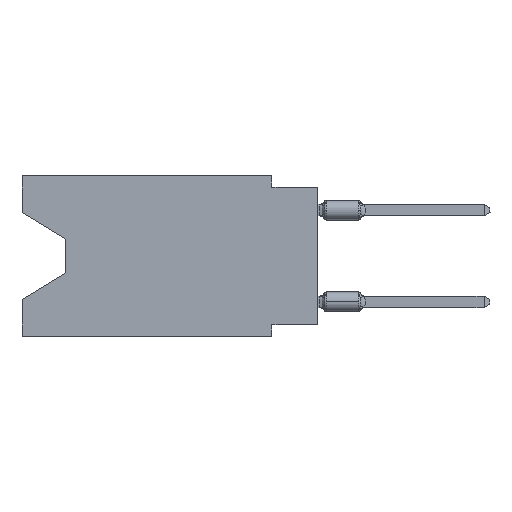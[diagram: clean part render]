
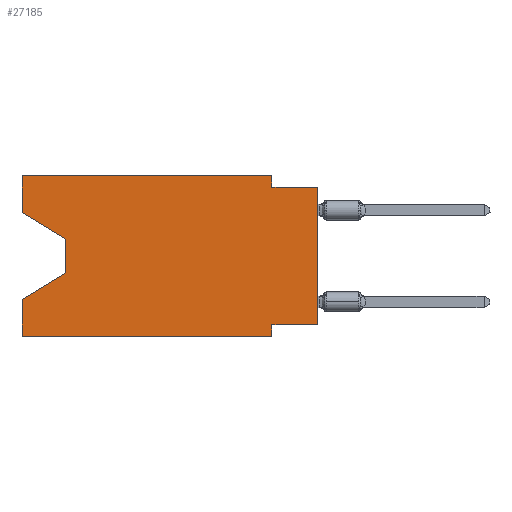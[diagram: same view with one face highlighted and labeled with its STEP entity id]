
A CAD part, left-side view. The second image highlights one B-rep face of the part: STEP entity #27185.
In plain terms, the highlighted planar face has unit normal (-1, 0, 0).
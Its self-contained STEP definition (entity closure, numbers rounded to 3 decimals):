
#173 = ORIENTED_EDGE ( 'NONE', *, *, #14531, .T. ) ;
#1053 = CARTESIAN_POINT ( 'NONE',  ( 0., 2.54, 0. ) ) ;
#1490 = CARTESIAN_POINT ( 'NONE',  ( 0., 16.383, -8.89 ) ) ;
#1505 = DIRECTION ( 'NONE',  ( 0., -1., 0. ) ) ;
#1600 = VERTEX_POINT ( 'NONE', #3688 ) ;
#1727 = ORIENTED_EDGE ( 'NONE', *, *, #35090, .T. ) ;
#1918 = CARTESIAN_POINT ( 'NONE',  ( 0., 2.54, -8.255 ) ) ;
#2110 = VERTEX_POINT ( 'NONE', #28559 ) ;
#2384 = VECTOR ( 'NONE', #1505, 1000. ) ;
#2463 = CARTESIAN_POINT ( 'NONE',  ( 0., 13.97, -5.385 ) ) ;
#3688 = CARTESIAN_POINT ( 'NONE',  ( 0., 13.97, -5.385 ) ) ;
#3735 = CARTESIAN_POINT ( 'NONE',  ( 0., 0., -0.635 ) ) ;
#5222 = LINE ( 'NONE', #19776, #11342 ) ;
#6176 = CARTESIAN_POINT ( 'NONE',  ( 0., 16.383, 0. ) ) ;
#6453 = VERTEX_POINT ( 'NONE', #34848 ) ;
#6454 = LINE ( 'NONE', #29892, #19715 ) ;
#6545 = DIRECTION ( 'NONE',  ( 0., 0., -1. ) ) ;
#6986 = ORIENTED_EDGE ( 'NONE', *, *, #32904, .F. ) ;
#8345 = VECTOR ( 'NONE', #33208, 1000. ) ;
#11218 = PLANE ( 'NONE',  #14468 ) ;
#11342 = VECTOR ( 'NONE', #28472, 1000. ) ;
#11491 = EDGE_CURVE ( 'NONE', #31974, #31664, #28038, .T. ) ;
#11546 = ORIENTED_EDGE ( 'NONE', *, *, #26068, .F. ) ;
#11664 = DIRECTION ( 'NONE',  ( 0., -1., 0. ) ) ;
#12173 = VERTEX_POINT ( 'NONE', #15195 ) ;
#12175 = CARTESIAN_POINT ( 'NONE',  ( 0., 2.54, -8.89 ) ) ;
#12543 = LINE ( 'NONE', #18385, #14503 ) ;
#13282 = DIRECTION ( 'NONE',  ( 0., 0., 1. ) ) ;
#13915 = VECTOR ( 'NONE', #13282, 1000. ) ;
#14278 = LINE ( 'NONE', #34992, #37591 ) ;
#14468 = AXIS2_PLACEMENT_3D ( 'NONE', #6176, #23044, #34839 ) ;
#14503 = VECTOR ( 'NONE', #6545, 1000. ) ;
#14531 = EDGE_CURVE ( 'NONE', #6453, #1600, #14278, .T. ) ;
#14732 = ORIENTED_EDGE ( 'NONE', *, *, #16717, .F. ) ;
#15039 = EDGE_CURVE ( 'NONE', #15574, #6453, #6454, .T. ) ;
#15195 = CARTESIAN_POINT ( 'NONE',  ( 0., 16.383, 0. ) ) ;
#15276 = LINE ( 'NONE', #16893, #19425 ) ;
#15574 = VERTEX_POINT ( 'NONE', #21343 ) ;
#15606 = DIRECTION ( 'NONE',  ( 0., 1., 0. ) ) ;
#16452 = ORIENTED_EDGE ( 'NONE', *, *, #33744, .F. ) ;
#16717 = EDGE_CURVE ( 'NONE', #12173, #18472, #32379, .T. ) ;
#16893 = CARTESIAN_POINT ( 'NONE',  ( 0., 0., -0.635 ) ) ;
#16964 = VECTOR ( 'NONE', #26086, 1000. ) ;
#17087 = VERTEX_POINT ( 'NONE', #25392 ) ;
#17481 = ORIENTED_EDGE ( 'NONE', *, *, #28936, .F. ) ;
#18075 = VECTOR ( 'NONE', #11664, 1000. ) ;
#18157 = CARTESIAN_POINT ( 'NONE',  ( 0., 0., -8.255 ) ) ;
#18254 = CARTESIAN_POINT ( 'NONE',  ( 0., 16.383, 0. ) ) ;
#18385 = CARTESIAN_POINT ( 'NONE',  ( 0., 2.54, -8.89 ) ) ;
#18472 = VERTEX_POINT ( 'NONE', #37056 ) ;
#19158 = CARTESIAN_POINT ( 'NONE',  ( 0., 16.383, -8.89 ) ) ;
#19425 = VECTOR ( 'NONE', #29795, 1000. ) ;
#19715 = VECTOR ( 'NONE', #32229, 1000. ) ;
#19776 = CARTESIAN_POINT ( 'NONE',  ( 0., 16.383, 0. ) ) ;
#21069 = LINE ( 'NONE', #18157, #28153 ) ;
#21343 = CARTESIAN_POINT ( 'NONE',  ( 0., 16.383, -2.038 ) ) ;
#21698 = ORIENTED_EDGE ( 'NONE', *, *, #27615, .T. ) ;
#21775 = LINE ( 'NONE', #1053, #8345 ) ;
#21845 = EDGE_CURVE ( 'NONE', #18472, #29876, #21775, .T. ) ;
#23044 = DIRECTION ( 'NONE',  ( 1., 0., 0. ) ) ;
#25213 = EDGE_CURVE ( 'NONE', #15574, #12173, #5222, .T. ) ;
#25392 = CARTESIAN_POINT ( 'NONE',  ( 0., 16.383, -6.852 ) ) ;
#25735 = LINE ( 'NONE', #28824, #30532 ) ;
#26068 = EDGE_CURVE ( 'NONE', #36453, #31664, #12543, .T. ) ;
#26086 = DIRECTION ( 'NONE',  ( 0., 0.855, -0.519 ) ) ;
#27185 = ADVANCED_FACE ( 'NONE', ( #32716 ), #11218, .F. ) ;
#27615 = EDGE_CURVE ( 'NONE', #1600, #17087, #31902, .T. ) ;
#27989 = CARTESIAN_POINT ( 'NONE',  ( 0., 16.383, 0. ) ) ;
#28038 = LINE ( 'NONE', #19158, #2384 ) ;
#28153 = VECTOR ( 'NONE', #15606, 1000. ) ;
#28188 = LINE ( 'NONE', #27989, #13915 ) ;
#28472 = DIRECTION ( 'NONE',  ( 0., 0., 1. ) ) ;
#28559 = CARTESIAN_POINT ( 'NONE',  ( 0., 0., -8.255 ) ) ;
#28719 = ORIENTED_EDGE ( 'NONE', *, *, #11491, .T. ) ;
#28824 = CARTESIAN_POINT ( 'NONE',  ( 0., 0., 0. ) ) ;
#28936 = EDGE_CURVE ( 'NONE', #2110, #36453, #21069, .T. ) ;
#29012 = DIRECTION ( 'NONE',  ( 0., 0., 1. ) ) ;
#29758 = EDGE_LOOP ( 'NONE', ( #30259, #173, #21698, #16452, #28719, #11546, #17481, #1727, #6986, #29855, #14732, #34719 ) ) ;
#29795 = DIRECTION ( 'NONE',  ( 0., -1., 0. ) ) ;
#29855 = ORIENTED_EDGE ( 'NONE', *, *, #21845, .F. ) ;
#29876 = VERTEX_POINT ( 'NONE', #37578 ) ;
#29892 = CARTESIAN_POINT ( 'NONE',  ( 0., 16.383, -2.038 ) ) ;
#30259 = ORIENTED_EDGE ( 'NONE', *, *, #15039, .T. ) ;
#30532 = VECTOR ( 'NONE', #29012, 1000. ) ;
#31664 = VERTEX_POINT ( 'NONE', #12175 ) ;
#31902 = LINE ( 'NONE', #2463, #16964 ) ;
#31974 = VERTEX_POINT ( 'NONE', #1490 ) ;
#32229 = DIRECTION ( 'NONE',  ( 0., -0.855, -0.519 ) ) ;
#32379 = LINE ( 'NONE', #18254, #18075 ) ;
#32644 = VERTEX_POINT ( 'NONE', #3735 ) ;
#32716 = FACE_OUTER_BOUND ( 'NONE', #29758, .T. ) ;
#32904 = EDGE_CURVE ( 'NONE', #29876, #32644, #15276, .T. ) ;
#33208 = DIRECTION ( 'NONE',  ( 0., 0., -1. ) ) ;
#33744 = EDGE_CURVE ( 'NONE', #31974, #17087, #28188, .T. ) ;
#34719 = ORIENTED_EDGE ( 'NONE', *, *, #25213, .F. ) ;
#34839 = DIRECTION ( 'NONE',  ( 0., 0., -1. ) ) ;
#34848 = CARTESIAN_POINT ( 'NONE',  ( 0., 13.97, -3.505 ) ) ;
#34992 = CARTESIAN_POINT ( 'NONE',  ( 0., 13.97, -3.505 ) ) ;
#35090 = EDGE_CURVE ( 'NONE', #2110, #32644, #25735, .T. ) ;
#36453 = VERTEX_POINT ( 'NONE', #1918 ) ;
#37056 = CARTESIAN_POINT ( 'NONE',  ( 0., 2.54, 0. ) ) ;
#37504 = DIRECTION ( 'NONE',  ( 0., 0., -1. ) ) ;
#37578 = CARTESIAN_POINT ( 'NONE',  ( 0., 2.54, -0.635 ) ) ;
#37591 = VECTOR ( 'NONE', #37504, 1000. ) ;
